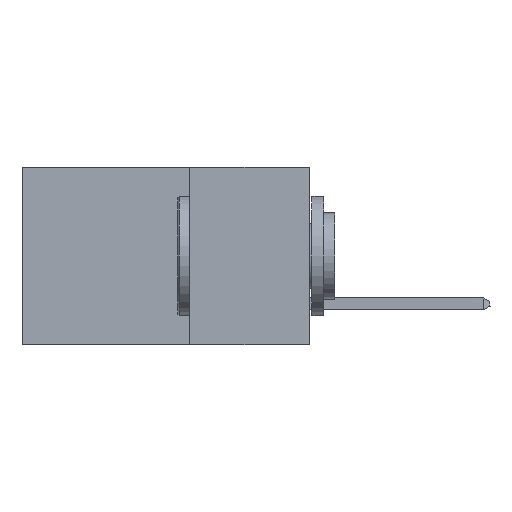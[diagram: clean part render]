
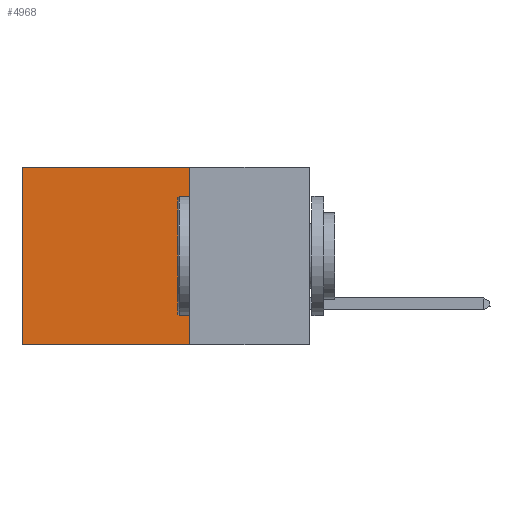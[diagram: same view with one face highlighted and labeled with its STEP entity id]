
A CAD part, left-side view. The second image highlights one B-rep face of the part: STEP entity #4968.
In plain terms, the highlighted planar face has unit normal (-1, 0, 0).
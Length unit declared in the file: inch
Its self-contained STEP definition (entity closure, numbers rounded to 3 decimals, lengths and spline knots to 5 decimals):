
#314 = CARTESIAN_POINT ( 'NONE',  ( 0.2875, 0.25, 0. ) ) ;
#1275 = CARTESIAN_POINT ( 'NONE',  ( 0.2875, 0.6, 0. ) ) ;
#1729 = CARTESIAN_POINT ( 'NONE',  ( 0.2875, 0.6, -0.37 ) ) ;
#2183 = DIRECTION ( 'NONE',  ( 0., 0., -1. ) ) ;
#2268 = VERTEX_POINT ( 'NONE', #13710 ) ;
#2612 = DIRECTION ( 'NONE',  ( 0., 0., -1. ) ) ;
#3000 = EDGE_CURVE ( 'NONE', #5295, #2268, #7552, .T. ) ;
#3619 = VECTOR ( 'NONE', #17526, 39.37008 ) ;
#3697 = CARTESIAN_POINT ( 'NONE',  ( 0.2875, 0.25, 0. ) ) ;
#3765 = DIRECTION ( 'NONE',  ( 0., 1., 0. ) ) ;
#3919 = VECTOR ( 'NONE', #2612, 39.37008 ) ;
#4968 = ADVANCED_FACE ( 'NONE', ( #8566 ), #10358, .F. ) ;
#5295 = VERTEX_POINT ( 'NONE', #18547 ) ;
#5397 = ORIENTED_EDGE ( 'NONE', *, *, #11587, .T. ) ;
#5707 = LINE ( 'NONE', #18608, #12879 ) ;
#6647 = ORIENTED_EDGE ( 'NONE', *, *, #16044, .F. ) ;
#7552 = LINE ( 'NONE', #3697, #10069 ) ;
#8399 = LINE ( 'NONE', #13130, #3619 ) ;
#8566 = FACE_OUTER_BOUND ( 'NONE', #16792, .T. ) ;
#9139 = EDGE_CURVE ( 'NONE', #15914, #16077, #5707, .T. ) ;
#9729 = ORIENTED_EDGE ( 'NONE', *, *, #9139, .F. ) ;
#9986 = DIRECTION ( 'NONE',  ( 0., 1., 0. ) ) ;
#10069 = VECTOR ( 'NONE', #3765, 39.37008 ) ;
#10358 = PLANE ( 'NONE',  #16127 ) ;
#11587 = EDGE_CURVE ( 'NONE', #2268, #16077, #11790, .T. ) ;
#11790 = LINE ( 'NONE', #1275, #3919 ) ;
#12879 = VECTOR ( 'NONE', #9986, 39.37008 ) ;
#13130 = CARTESIAN_POINT ( 'NONE',  ( 0.2875, 0.25, 0. ) ) ;
#13632 = DIRECTION ( 'NONE',  ( 1., 0., 0. ) ) ;
#13710 = CARTESIAN_POINT ( 'NONE',  ( 0.2875, 0.6, 0. ) ) ;
#15260 = ORIENTED_EDGE ( 'NONE', *, *, #3000, .T. ) ;
#15914 = VERTEX_POINT ( 'NONE', #16918 ) ;
#16044 = EDGE_CURVE ( 'NONE', #5295, #15914, #8399, .T. ) ;
#16077 = VERTEX_POINT ( 'NONE', #1729 ) ;
#16127 = AXIS2_PLACEMENT_3D ( 'NONE', #314, #13632, #2183 ) ;
#16792 = EDGE_LOOP ( 'NONE', ( #5397, #9729, #6647, #15260 ) ) ;
#16918 = CARTESIAN_POINT ( 'NONE',  ( 0.2875, 0.25, -0.37 ) ) ;
#17526 = DIRECTION ( 'NONE',  ( 0., 0., -1. ) ) ;
#18547 = CARTESIAN_POINT ( 'NONE',  ( 0.2875, 0.25, 0. ) ) ;
#18608 = CARTESIAN_POINT ( 'NONE',  ( 0.2875, 0.25, -0.37 ) ) ;
